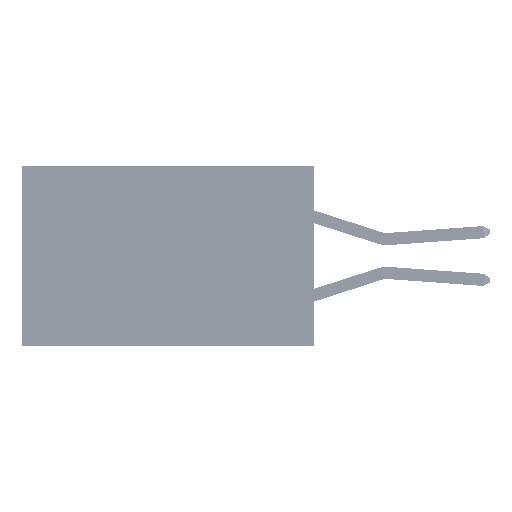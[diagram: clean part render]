
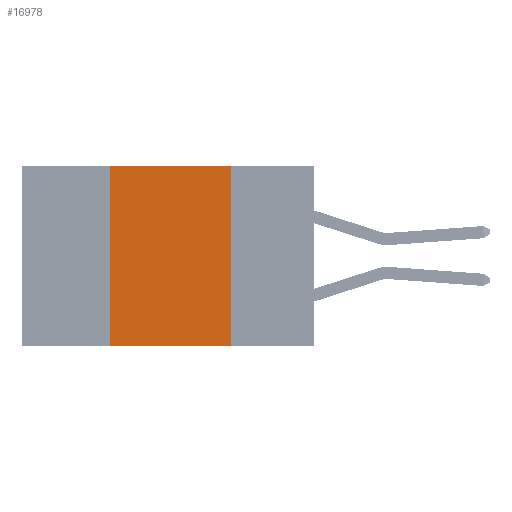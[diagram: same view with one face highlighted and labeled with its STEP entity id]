
A CAD part, left-side view. The second image highlights one B-rep face of the part: STEP entity #16978.
In plain terms, the highlighted planar face has unit normal (-1, 0, 0).
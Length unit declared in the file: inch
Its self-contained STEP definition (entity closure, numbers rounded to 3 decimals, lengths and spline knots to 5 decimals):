
#258 = ORIENTED_EDGE ( 'NONE', *, *, #24586, .T. ) ;
#326 = VECTOR ( 'NONE', #24398, 39.37008 ) ;
#1527 = ORIENTED_EDGE ( 'NONE', *, *, #34878, .F. ) ;
#2234 = VERTEX_POINT ( 'NONE', #33986 ) ;
#2248 = ORIENTED_EDGE ( 'NONE', *, *, #47169, .F. ) ;
#2449 = VERTEX_POINT ( 'NONE', #6368 ) ;
#3830 = LINE ( 'NONE', #31860, #326 ) ;
#4739 = LINE ( 'NONE', #9440, #43132 ) ;
#5557 = FACE_OUTER_BOUND ( 'NONE', #5616, .T. ) ;
#5616 = EDGE_LOOP ( 'NONE', ( #1527, #2248, #6602, #258 ) ) ;
#6368 = CARTESIAN_POINT ( 'NONE',  ( 0., 0.17, 0. ) ) ;
#6602 = ORIENTED_EDGE ( 'NONE', *, *, #35414, .F. ) ;
#9440 = CARTESIAN_POINT ( 'NONE',  ( 0., 0.6, 0. ) ) ;
#13164 = PLANE ( 'NONE',  #28614 ) ;
#13648 = CARTESIAN_POINT ( 'NONE',  ( 0., 0.6, 0. ) ) ;
#13930 = DIRECTION ( 'NONE',  ( 0., -1., 0. ) ) ;
#16779 = VECTOR ( 'NONE', #13930, 39.37008 ) ;
#16978 = ADVANCED_FACE ( 'NONE', ( #5557 ), #13164, .F. ) ;
#17139 = VERTEX_POINT ( 'NONE', #32648 ) ;
#19648 = CARTESIAN_POINT ( 'NONE',  ( 0., 0.42, 0. ) ) ;
#20275 = DIRECTION ( 'NONE',  ( 0., 0., 1. ) ) ;
#20962 = DIRECTION ( 'NONE',  ( 0., 0., -1. ) ) ;
#24398 = DIRECTION ( 'NONE',  ( 0., 0., -1. ) ) ;
#24586 = EDGE_CURVE ( 'NONE', #2234, #42832, #30711, .T. ) ;
#27822 = DIRECTION ( 'NONE',  ( 0., -1., 0. ) ) ;
#28614 = AXIS2_PLACEMENT_3D ( 'NONE', #13648, #46463, #20962 ) ;
#28710 = CARTESIAN_POINT ( 'NONE',  ( 0., 0.6, -0.37 ) ) ;
#30711 = LINE ( 'NONE', #28710, #16779 ) ;
#31860 = CARTESIAN_POINT ( 'NONE',  ( 0., 0.17, 0. ) ) ;
#32648 = CARTESIAN_POINT ( 'NONE',  ( 0., 0.42, 0. ) ) ;
#33986 = CARTESIAN_POINT ( 'NONE',  ( 0., 0.42, -0.37 ) ) ;
#34878 = EDGE_CURVE ( 'NONE', #2449, #42832, #3830, .T. ) ;
#35414 = EDGE_CURVE ( 'NONE', #2234, #17139, #43910, .T. ) ;
#42832 = VERTEX_POINT ( 'NONE', #42993 ) ;
#42993 = CARTESIAN_POINT ( 'NONE',  ( 0., 0.17, -0.37 ) ) ;
#43132 = VECTOR ( 'NONE', #27822, 39.37008 ) ;
#43910 = LINE ( 'NONE', #19648, #47936 ) ;
#46463 = DIRECTION ( 'NONE',  ( 1., 0., 0. ) ) ;
#47169 = EDGE_CURVE ( 'NONE', #17139, #2449, #4739, .T. ) ;
#47936 = VECTOR ( 'NONE', #20275, 39.37008 ) ;
